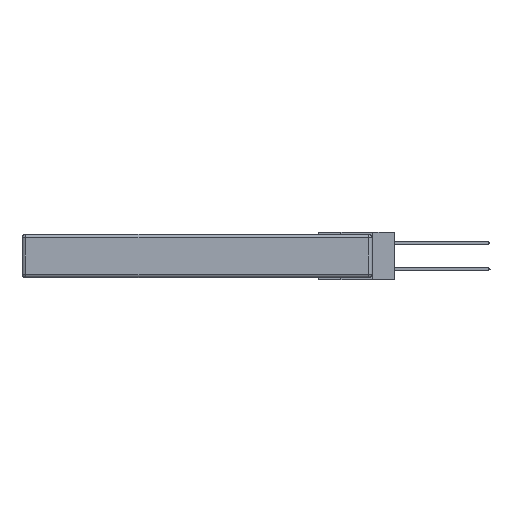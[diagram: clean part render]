
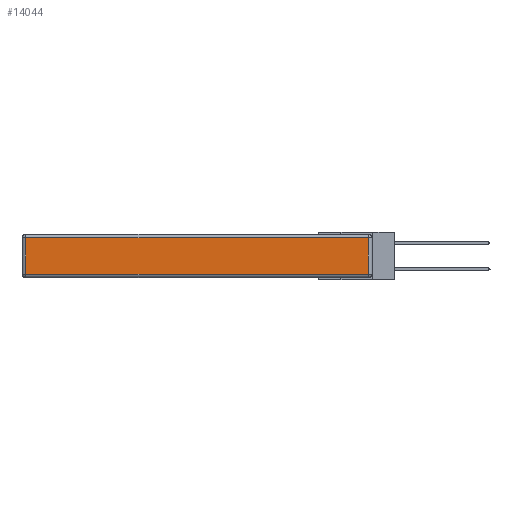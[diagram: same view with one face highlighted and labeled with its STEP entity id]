
A CAD part, left-side view. The second image highlights one B-rep face of the part: STEP entity #14044.
In plain terms, the highlighted planar face has unit normal (-1, 0, 0).
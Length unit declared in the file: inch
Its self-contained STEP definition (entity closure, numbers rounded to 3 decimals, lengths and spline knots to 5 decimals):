
#214 = VERTEX_POINT ( 'NONE', #32469 ) ;
#930 = EDGE_LOOP ( 'NONE', ( #33617, #24171, #8652, #31402 ) ) ;
#2220 = DIRECTION ( 'NONE',  ( 0., 1., 0. ) ) ;
#2367 = CARTESIAN_POINT ( 'NONE',  ( 0., 0., -0.313 ) ) ;
#2639 = CARTESIAN_POINT ( 'NONE',  ( 0., 2.72, -0.313 ) ) ;
#2705 = VECTOR ( 'NONE', #2220, 39.37008 ) ;
#3837 = AXIS2_PLACEMENT_3D ( 'NONE', #6810, #22295, #22529 ) ;
#5064 = CARTESIAN_POINT ( 'NONE',  ( 0., 2.75, -0.03 ) ) ;
#6810 = CARTESIAN_POINT ( 'NONE',  ( 0., 0., -0.343 ) ) ;
#8009 = CARTESIAN_POINT ( 'NONE',  ( 0., 0.03, -0.343 ) ) ;
#8652 = ORIENTED_EDGE ( 'NONE', *, *, #20213, .T. ) ;
#9323 = CARTESIAN_POINT ( 'NONE',  ( 0., 2.72, -0.03 ) ) ;
#10500 = LINE ( 'NONE', #2367, #13786 ) ;
#12547 = VECTOR ( 'NONE', #21309, 39.37008 ) ;
#12931 = LINE ( 'NONE', #8009, #12547 ) ;
#13786 = VECTOR ( 'NONE', #25656, 39.37008 ) ;
#14044 = ADVANCED_FACE ( 'NONE', ( #31305 ), #30351, .T. ) ;
#16044 = DIRECTION ( 'NONE',  ( 0., 0., -1. ) ) ;
#16681 = VERTEX_POINT ( 'NONE', #19416 ) ;
#19416 = CARTESIAN_POINT ( 'NONE',  ( 0., 0.03, -0.03 ) ) ;
#19797 = EDGE_CURVE ( 'NONE', #25308, #214, #10500, .T. ) ;
#20213 = EDGE_CURVE ( 'NONE', #16681, #28278, #21564, .T. ) ;
#20259 = EDGE_CURVE ( 'NONE', #214, #16681, #12931, .T. ) ;
#21309 = DIRECTION ( 'NONE',  ( 0., 0., 1. ) ) ;
#21564 = LINE ( 'NONE', #5064, #2705 ) ;
#22153 = VECTOR ( 'NONE', #16044, 39.37008 ) ;
#22295 = DIRECTION ( 'NONE',  ( -1., 0., 0. ) ) ;
#22529 = DIRECTION ( 'NONE',  ( 0., 0., 1. ) ) ;
#24171 = ORIENTED_EDGE ( 'NONE', *, *, #20259, .T. ) ;
#25308 = VERTEX_POINT ( 'NONE', #2639 ) ;
#25656 = DIRECTION ( 'NONE',  ( 0., -1., 0. ) ) ;
#26185 = EDGE_CURVE ( 'NONE', #28278, #25308, #27100, .T. ) ;
#27100 = LINE ( 'NONE', #31785, #22153 ) ;
#28278 = VERTEX_POINT ( 'NONE', #9323 ) ;
#30351 = PLANE ( 'NONE',  #3837 ) ;
#31305 = FACE_OUTER_BOUND ( 'NONE', #930, .T. ) ;
#31402 = ORIENTED_EDGE ( 'NONE', *, *, #26185, .T. ) ;
#31785 = CARTESIAN_POINT ( 'NONE',  ( 0., 2.72, -0.343 ) ) ;
#32469 = CARTESIAN_POINT ( 'NONE',  ( 0., 0.03, -0.313 ) ) ;
#33617 = ORIENTED_EDGE ( 'NONE', *, *, #19797, .T. ) ;
